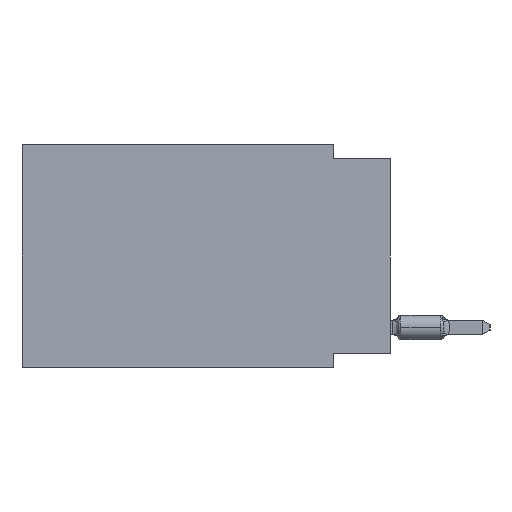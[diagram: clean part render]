
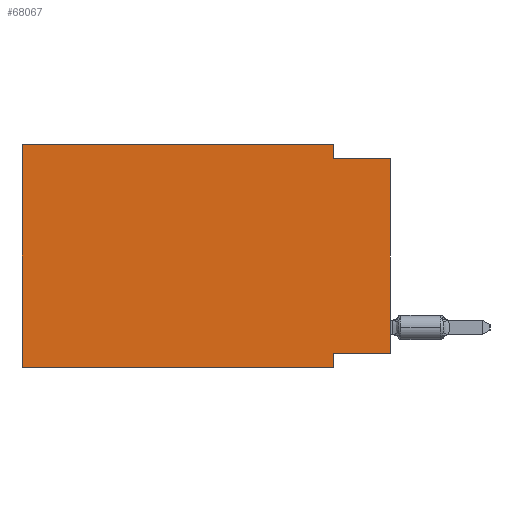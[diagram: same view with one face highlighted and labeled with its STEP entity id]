
A CAD part, left-side view. The second image highlights one B-rep face of the part: STEP entity #68067.
In plain terms, the highlighted planar face has unit normal (-1, 0, 0).
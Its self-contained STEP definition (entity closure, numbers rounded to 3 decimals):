
#242 = LINE ( 'NONE', #10964, #29351 ) ;
#959 = DIRECTION ( 'NONE',  ( 0., 1., 0. ) ) ;
#1505 = CARTESIAN_POINT ( 'NONE',  ( 0., 16.383, 0. ) ) ;
#1992 = EDGE_CURVE ( 'NONE', #63190, #24341, #56076, .T. ) ;
#2838 = CARTESIAN_POINT ( 'NONE',  ( 0., 16.383, -9.906 ) ) ;
#4450 = ORIENTED_EDGE ( 'NONE', *, *, #56485, .F. ) ;
#6960 = ORIENTED_EDGE ( 'NONE', *, *, #30310, .T. ) ;
#7230 = ORIENTED_EDGE ( 'NONE', *, *, #1992, .F. ) ;
#8206 = CARTESIAN_POINT ( 'NONE',  ( 0., 0., 0. ) ) ;
#8585 = DIRECTION ( 'NONE',  ( 0., 0., 1. ) ) ;
#8650 = DIRECTION ( 'NONE',  ( 0., 0., -1. ) ) ;
#10283 = DIRECTION ( 'NONE',  ( 0., -1., 0. ) ) ;
#10558 = VERTEX_POINT ( 'NONE', #2838 ) ;
#10964 = CARTESIAN_POINT ( 'NONE',  ( 0., 0., -9.271 ) ) ;
#13831 = VERTEX_POINT ( 'NONE', #59576 ) ;
#15944 = FACE_OUTER_BOUND ( 'NONE', #42160, .T. ) ;
#17634 = CARTESIAN_POINT ( 'NONE',  ( 0., 0., -0.635 ) ) ;
#17664 = VECTOR ( 'NONE', #10283, 1000. ) ;
#20377 = LINE ( 'NONE', #59884, #30113 ) ;
#20775 = ORIENTED_EDGE ( 'NONE', *, *, #43021, .F. ) ;
#21116 = DIRECTION ( 'NONE',  ( 1., 0., 0. ) ) ;
#21493 = PLANE ( 'NONE',  #21606 ) ;
#21606 = AXIS2_PLACEMENT_3D ( 'NONE', #60275, #21116, #27014 ) ;
#23683 = LINE ( 'NONE', #1505, #71125 ) ;
#23744 = CARTESIAN_POINT ( 'NONE',  ( 0., 16.383, 0. ) ) ;
#24341 = VERTEX_POINT ( 'NONE', #55632 ) ;
#24435 = ORIENTED_EDGE ( 'NONE', *, *, #72359, .T. ) ;
#27014 = DIRECTION ( 'NONE',  ( 0., 0., -1. ) ) ;
#27756 = CARTESIAN_POINT ( 'NONE',  ( 0., 2.54, 0. ) ) ;
#29351 = VECTOR ( 'NONE', #959, 1000. ) ;
#30113 = VECTOR ( 'NONE', #42525, 1000. ) ;
#30310 = EDGE_CURVE ( 'NONE', #13831, #24341, #36673, .T. ) ;
#31042 = VECTOR ( 'NONE', #56102, 1000. ) ;
#31411 = EDGE_CURVE ( 'NONE', #13831, #66969, #242, .T. ) ;
#31594 = VERTEX_POINT ( 'NONE', #63738 ) ;
#31649 = ORIENTED_EDGE ( 'NONE', *, *, #31411, .F. ) ;
#33359 = VERTEX_POINT ( 'NONE', #23744 ) ;
#34297 = EDGE_CURVE ( 'NONE', #66969, #31594, #70347, .T. ) ;
#36673 = LINE ( 'NONE', #8206, #37683 ) ;
#36720 = CARTESIAN_POINT ( 'NONE',  ( 0., 2.54, -9.271 ) ) ;
#37683 = VECTOR ( 'NONE', #8585, 1000. ) ;
#41763 = DIRECTION ( 'NONE',  ( 0., -1., 0. ) ) ;
#42160 = EDGE_LOOP ( 'NONE', ( #6960, #7230, #20775, #4450, #51235, #24435, #72582, #31649 ) ) ;
#42525 = DIRECTION ( 'NONE',  ( 0., -1., 0. ) ) ;
#43021 = EDGE_CURVE ( 'NONE', #55706, #63190, #61730, .T. ) ;
#43459 = EDGE_CURVE ( 'NONE', #10558, #33359, #61267, .T. ) ;
#49191 = DIRECTION ( 'NONE',  ( 0., 0., -1. ) ) ;
#51235 = ORIENTED_EDGE ( 'NONE', *, *, #43459, .F. ) ;
#51240 = CARTESIAN_POINT ( 'NONE',  ( 0., 2.54, -0.635 ) ) ;
#55632 = CARTESIAN_POINT ( 'NONE',  ( 0., 0., -0.635 ) ) ;
#55706 = VERTEX_POINT ( 'NONE', #69489 ) ;
#56076 = LINE ( 'NONE', #17634, #17664 ) ;
#56102 = DIRECTION ( 'NONE',  ( 0., 0., 1. ) ) ;
#56485 = EDGE_CURVE ( 'NONE', #33359, #55706, #23683, .T. ) ;
#59576 = CARTESIAN_POINT ( 'NONE',  ( 0., 0., -9.271 ) ) ;
#59884 = CARTESIAN_POINT ( 'NONE',  ( 0., 16.383, -9.906 ) ) ;
#60275 = CARTESIAN_POINT ( 'NONE',  ( 0., 16.383, 0. ) ) ;
#60367 = CARTESIAN_POINT ( 'NONE',  ( 0., 2.54, -9.906 ) ) ;
#61267 = LINE ( 'NONE', #71997, #31042 ) ;
#61730 = LINE ( 'NONE', #27756, #66382 ) ;
#63190 = VERTEX_POINT ( 'NONE', #51240 ) ;
#63738 = CARTESIAN_POINT ( 'NONE',  ( 0., 2.54, -9.906 ) ) ;
#65055 = VECTOR ( 'NONE', #8650, 1000. ) ;
#66382 = VECTOR ( 'NONE', #49191, 1000. ) ;
#66969 = VERTEX_POINT ( 'NONE', #36720 ) ;
#68067 = ADVANCED_FACE ( 'NONE', ( #15944 ), #21493, .F. ) ;
#69489 = CARTESIAN_POINT ( 'NONE',  ( 0., 2.54, 0. ) ) ;
#70347 = LINE ( 'NONE', #60367, #65055 ) ;
#71125 = VECTOR ( 'NONE', #41763, 1000. ) ;
#71997 = CARTESIAN_POINT ( 'NONE',  ( 0., 16.383, 0. ) ) ;
#72359 = EDGE_CURVE ( 'NONE', #10558, #31594, #20377, .T. ) ;
#72582 = ORIENTED_EDGE ( 'NONE', *, *, #34297, .F. ) ;
